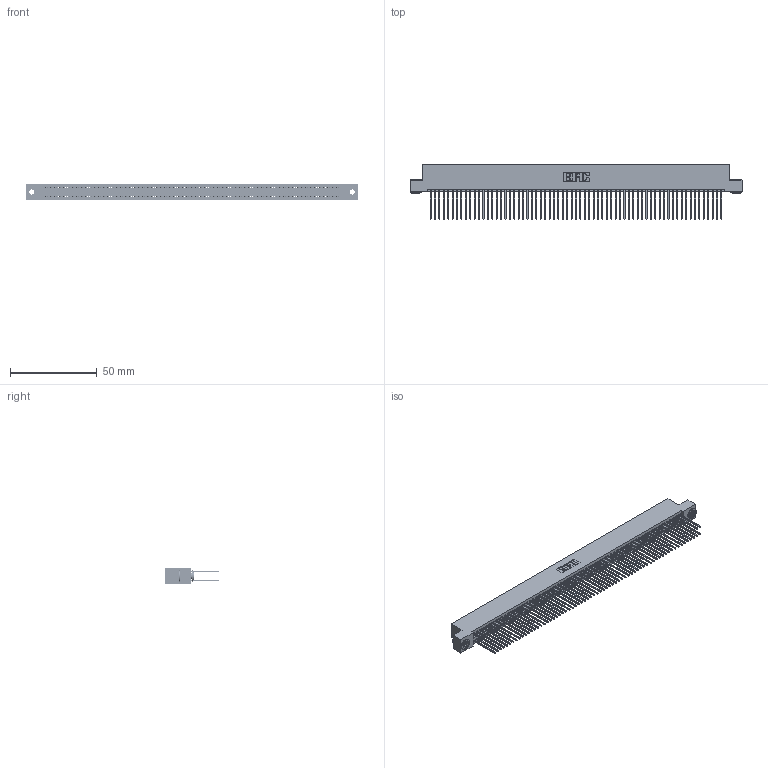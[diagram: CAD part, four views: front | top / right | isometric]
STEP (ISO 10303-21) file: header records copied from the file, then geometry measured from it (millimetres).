
FILE_DESCRIPTION (( 'STEP AP203' ), '1' );
FILE_NAME ('345-134-542-203.STEP', '2019-11-08T02:44:02', ( '' ), ( '' ), 'SwSTEP 2.0', 'SolidWorks 2016', '' );
FILE_SCHEMA (( 'CONFIG_CONTROL_DESIGN' ));
Length unit declared in the file: inch
Products named in the file (4): 345 Part_Flush Mounting Lugs - 0.156 Dia-TH; 345-134-542-203; 345-250-002_345-250-002-102; 345-292-001_345-293-142
Assembly tree (137 placements, depth 2):
  345-134-542-203
    345 Part_Flush Mounting Lugs - 0.156 Dia-TH
    345-292-001_345-293-142  x134
    345-250-002_345-250-002-102  x2
Bounding box: 191.39 x 31.29 x 9.4 mm (x, y, z)
Volume: 19467.8 mm3; surface area: 32385 mm2
Topology: 137 solids, 137 shells, 6864 faces, 20383 edges, 13406 vertices
Faces by surface type: plane 4512, cylinder 2344, cone 8
Entity records: 49872 total; most frequent: CARTESIAN_POINT 8311, ORIENTED_EDGE 8238, DIRECTION 7329, EDGE_CURVE 4119, LINE 3695, VECTOR 3695, VERTEX_POINT 2742, AXIS2_PLACEMENT_3D 1817
